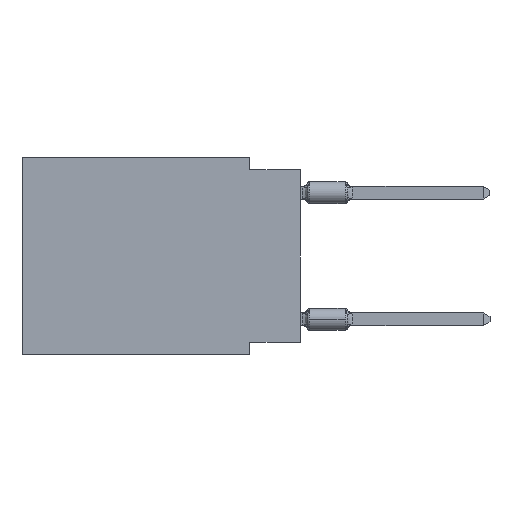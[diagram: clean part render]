
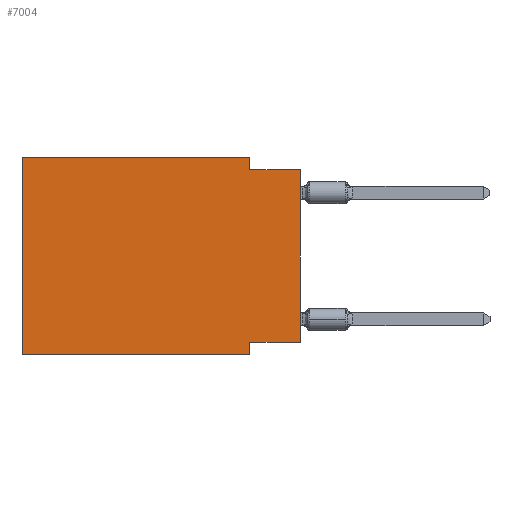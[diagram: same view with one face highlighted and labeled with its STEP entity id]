
A CAD part, left-side view. The second image highlights one B-rep face of the part: STEP entity #7004.
In plain terms, the highlighted planar face has unit normal (-1, 0, 0).
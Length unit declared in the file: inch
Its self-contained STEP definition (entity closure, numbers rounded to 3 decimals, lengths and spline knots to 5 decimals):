
#95 = VERTEX_POINT ( 'NONE', #13392 ) ;
#410 = DIRECTION ( 'NONE',  ( 0., -1., 0. ) ) ;
#413 = CARTESIAN_POINT ( 'NONE',  ( 0., 0., 0. ) ) ;
#558 = CARTESIAN_POINT ( 'NONE',  ( 0., 0.55, -0.39 ) ) ;
#949 = CARTESIAN_POINT ( 'NONE',  ( 0., 0.1, -0.39 ) ) ;
#955 = CARTESIAN_POINT ( 'NONE',  ( 0., 0.55, 0. ) ) ;
#1085 = CARTESIAN_POINT ( 'NONE',  ( 0., 0., -0.365 ) ) ;
#1247 = DIRECTION ( 'NONE',  ( 0., 0., -1. ) ) ;
#1338 = CARTESIAN_POINT ( 'NONE',  ( 0., 0.1, 0. ) ) ;
#1923 = EDGE_CURVE ( 'NONE', #16344, #10768, #12550, .T. ) ;
#3435 = CARTESIAN_POINT ( 'NONE',  ( 0., 0.1, -0.025 ) ) ;
#3620 = ORIENTED_EDGE ( 'NONE', *, *, #8927, .T. ) ;
#3691 = ORIENTED_EDGE ( 'NONE', *, *, #5223, .F. ) ;
#4208 = VERTEX_POINT ( 'NONE', #11784 ) ;
#4279 = DIRECTION ( 'NONE',  ( 0., -1., 0. ) ) ;
#4381 = CARTESIAN_POINT ( 'NONE',  ( 0., 0., -0.025 ) ) ;
#4528 = LINE ( 'NONE', #949, #7327 ) ;
#5223 = EDGE_CURVE ( 'NONE', #19391, #4208, #11205, .T. ) ;
#5601 = LINE ( 'NONE', #955, #7258 ) ;
#5690 = VECTOR ( 'NONE', #6812, 39.37008 ) ;
#5766 = EDGE_LOOP ( 'NONE', ( #12644, #19332, #19884, #17456, #18153, #3620, #9119, #3691 ) ) ;
#5881 = EDGE_CURVE ( 'NONE', #95, #16344, #5601, .T. ) ;
#5919 = DIRECTION ( 'NONE',  ( 0., 0., 1. ) ) ;
#6110 = DIRECTION ( 'NONE',  ( 0., 0., -1. ) ) ;
#6198 = VECTOR ( 'NONE', #6110, 39.37008 ) ;
#6583 = LINE ( 'NONE', #14246, #17346 ) ;
#6812 = DIRECTION ( 'NONE',  ( 0., -1., 0. ) ) ;
#7004 = ADVANCED_FACE ( 'NONE', ( #7033 ), #8553, .F. ) ;
#7033 = FACE_OUTER_BOUND ( 'NONE', #5766, .T. ) ;
#7258 = VECTOR ( 'NONE', #4279, 39.37008 ) ;
#7302 = EDGE_CURVE ( 'NONE', #10768, #10112, #11246, .T. ) ;
#7327 = VECTOR ( 'NONE', #10131, 39.37008 ) ;
#7435 = LINE ( 'NONE', #18344, #15105 ) ;
#7690 = CARTESIAN_POINT ( 'NONE',  ( 0., 0.1, 0. ) ) ;
#8039 = CARTESIAN_POINT ( 'NONE',  ( 0., 0., -0.025 ) ) ;
#8184 = VERTEX_POINT ( 'NONE', #10072 ) ;
#8417 = LINE ( 'NONE', #413, #11758 ) ;
#8553 = PLANE ( 'NONE',  #13083 ) ;
#8927 = EDGE_CURVE ( 'NONE', #15584, #8184, #6583, .T. ) ;
#9119 = ORIENTED_EDGE ( 'NONE', *, *, #15541, .F. ) ;
#9488 = CARTESIAN_POINT ( 'NONE',  ( 0., 0., -0.365 ) ) ;
#10072 = CARTESIAN_POINT ( 'NONE',  ( 0., 0.1, -0.39 ) ) ;
#10112 = VERTEX_POINT ( 'NONE', #4381 ) ;
#10131 = DIRECTION ( 'NONE',  ( 0., 0., -1. ) ) ;
#10768 = VERTEX_POINT ( 'NONE', #3435 ) ;
#11205 = LINE ( 'NONE', #9488, #13677 ) ;
#11246 = LINE ( 'NONE', #8039, #5690 ) ;
#11319 = DIRECTION ( 'NONE',  ( 0., 0., 1. ) ) ;
#11438 = EDGE_CURVE ( 'NONE', #15584, #95, #7435, .T. ) ;
#11758 = VECTOR ( 'NONE', #11319, 39.37008 ) ;
#11784 = CARTESIAN_POINT ( 'NONE',  ( 0., 0.1, -0.365 ) ) ;
#12550 = LINE ( 'NONE', #1338, #6198 ) ;
#12644 = ORIENTED_EDGE ( 'NONE', *, *, #13553, .T. ) ;
#13083 = AXIS2_PLACEMENT_3D ( 'NONE', #14990, #14803, #1247 ) ;
#13392 = CARTESIAN_POINT ( 'NONE',  ( 0., 0.55, 0. ) ) ;
#13553 = EDGE_CURVE ( 'NONE', #19391, #10112, #8417, .T. ) ;
#13677 = VECTOR ( 'NONE', #15635, 39.37008 ) ;
#14246 = CARTESIAN_POINT ( 'NONE',  ( 0., 0.55, -0.39 ) ) ;
#14803 = DIRECTION ( 'NONE',  ( 1., 0., 0. ) ) ;
#14990 = CARTESIAN_POINT ( 'NONE',  ( 0., 0.55, 0. ) ) ;
#15105 = VECTOR ( 'NONE', #5919, 39.37008 ) ;
#15541 = EDGE_CURVE ( 'NONE', #4208, #8184, #4528, .T. ) ;
#15584 = VERTEX_POINT ( 'NONE', #558 ) ;
#15635 = DIRECTION ( 'NONE',  ( 0., 1., 0. ) ) ;
#16344 = VERTEX_POINT ( 'NONE', #7690 ) ;
#17346 = VECTOR ( 'NONE', #410, 39.37008 ) ;
#17456 = ORIENTED_EDGE ( 'NONE', *, *, #5881, .F. ) ;
#18153 = ORIENTED_EDGE ( 'NONE', *, *, #11438, .F. ) ;
#18344 = CARTESIAN_POINT ( 'NONE',  ( 0., 0.55, 0. ) ) ;
#19332 = ORIENTED_EDGE ( 'NONE', *, *, #7302, .F. ) ;
#19391 = VERTEX_POINT ( 'NONE', #1085 ) ;
#19884 = ORIENTED_EDGE ( 'NONE', *, *, #1923, .F. ) ;
